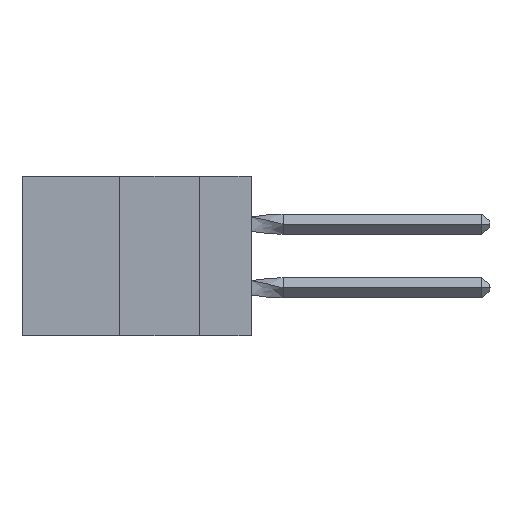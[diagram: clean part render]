
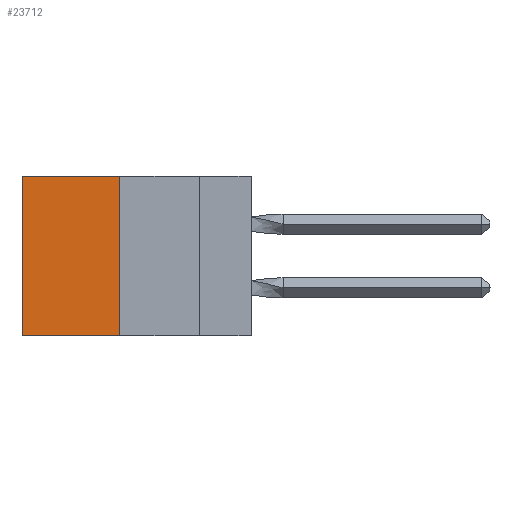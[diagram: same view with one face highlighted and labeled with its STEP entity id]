
A CAD part, left-side view. The second image highlights one B-rep face of the part: STEP entity #23712.
In plain terms, the highlighted planar face has unit normal (-1, 0, 0).
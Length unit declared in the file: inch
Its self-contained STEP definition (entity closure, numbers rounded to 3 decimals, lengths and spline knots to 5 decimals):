
#2071 = VECTOR ( 'NONE', #20197, 39.37008 ) ;
#4236 = EDGE_LOOP ( 'NONE', ( #18339, #13787, #16396, #26824 ) ) ;
#5410 = DIRECTION ( 'NONE',  ( 0., 0., -1. ) ) ;
#5930 = EDGE_CURVE ( 'NONE', #13302, #7131, #34382, .T. ) ;
#6047 = CARTESIAN_POINT ( 'NONE',  ( 0.305, 0.72, -0.5 ) ) ;
#6431 = LINE ( 'NONE', #6047, #2071 ) ;
#7131 = VERTEX_POINT ( 'NONE', #25454 ) ;
#8588 = DIRECTION ( 'NONE',  ( 1., 0., 0. ) ) ;
#8717 = CARTESIAN_POINT ( 'NONE',  ( 0.305, 0.413, -0.5 ) ) ;
#11180 = EDGE_CURVE ( 'NONE', #20046, #33209, #6431, .T. ) ;
#13302 = VERTEX_POINT ( 'NONE', #20934 ) ;
#13787 = ORIENTED_EDGE ( 'NONE', *, *, #32017, .F. ) ;
#15403 = CARTESIAN_POINT ( 'NONE',  ( 0.305, 0.72, 0. ) ) ;
#16396 = ORIENTED_EDGE ( 'NONE', *, *, #5930, .F. ) ;
#18339 = ORIENTED_EDGE ( 'NONE', *, *, #11180, .T. ) ;
#19751 = AXIS2_PLACEMENT_3D ( 'NONE', #8717, #8588, #5410 ) ;
#20046 = VERTEX_POINT ( 'NONE', #15403 ) ;
#20197 = DIRECTION ( 'NONE',  ( 0., 0., -1. ) ) ;
#20934 = CARTESIAN_POINT ( 'NONE',  ( 0.305, 0.413, 0. ) ) ;
#21212 = LINE ( 'NONE', #21550, #24650 ) ;
#21550 = CARTESIAN_POINT ( 'NONE',  ( 0.305, 0.413, 0. ) ) ;
#23301 = LINE ( 'NONE', #31333, #27655 ) ;
#23712 = ADVANCED_FACE ( 'NONE', ( #28856 ), #25153, .F. ) ;
#24210 = DIRECTION ( 'NONE',  ( 0., 1., 0. ) ) ;
#24650 = VECTOR ( 'NONE', #24210, 39.37008 ) ;
#25153 = PLANE ( 'NONE',  #19751 ) ;
#25454 = CARTESIAN_POINT ( 'NONE',  ( 0.305, 0.413, -0.5 ) ) ;
#26736 = CARTESIAN_POINT ( 'NONE',  ( 0.305, 0.413, -0.5 ) ) ;
#26824 = ORIENTED_EDGE ( 'NONE', *, *, #31607, .T. ) ;
#27655 = VECTOR ( 'NONE', #28439, 39.37008 ) ;
#28364 = VECTOR ( 'NONE', #29633, 39.37008 ) ;
#28439 = DIRECTION ( 'NONE',  ( 0., 1., 0. ) ) ;
#28856 = FACE_OUTER_BOUND ( 'NONE', #4236, .T. ) ;
#29633 = DIRECTION ( 'NONE',  ( 0., 0., -1. ) ) ;
#31333 = CARTESIAN_POINT ( 'NONE',  ( 0.305, 0.413, -0.5 ) ) ;
#31607 = EDGE_CURVE ( 'NONE', #13302, #20046, #21212, .T. ) ;
#32017 = EDGE_CURVE ( 'NONE', #7131, #33209, #23301, .T. ) ;
#33209 = VERTEX_POINT ( 'NONE', #33685 ) ;
#33685 = CARTESIAN_POINT ( 'NONE',  ( 0.305, 0.72, -0.5 ) ) ;
#34382 = LINE ( 'NONE', #26736, #28364 ) ;
